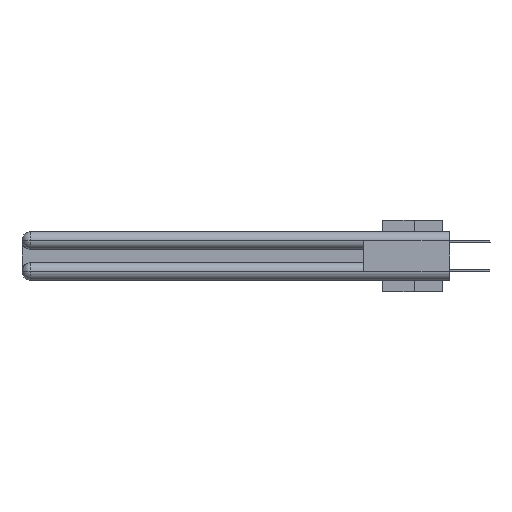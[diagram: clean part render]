
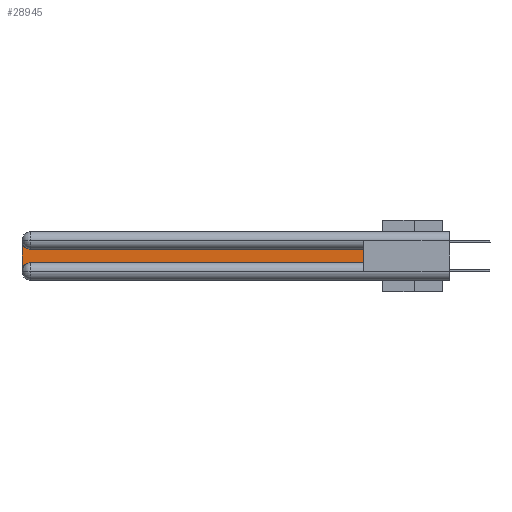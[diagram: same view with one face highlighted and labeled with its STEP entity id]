
A CAD part, left-side view. The second image highlights one B-rep face of the part: STEP entity #28945.
In plain terms, the highlighted planar face has unit normal (-1, 0, 0).
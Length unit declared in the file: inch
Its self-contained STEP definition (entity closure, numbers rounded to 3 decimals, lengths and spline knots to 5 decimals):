
#2207 = CARTESIAN_POINT ( 'NONE',  ( 0.075, 0.6, -0.2175 ) ) ;
#2343 = LINE ( 'NONE', #18107, #22983 ) ;
#2412 = CARTESIAN_POINT ( 'NONE',  ( 0.075, 3., -0.2175 ) ) ;
#2614 = LINE ( 'NONE', #2412, #15412 ) ;
#3167 = VERTEX_POINT ( 'NONE', #26577 ) ;
#3244 = ORIENTED_EDGE ( 'NONE', *, *, #26039, .T. ) ;
#3296 = AXIS2_PLACEMENT_3D ( 'NONE', #23964, #34139, #24758 ) ;
#4093 = CARTESIAN_POINT ( 'NONE',  ( 0.075, 2.94, -0.2775 ) ) ;
#6025 = DIRECTION ( 'NONE',  ( 0., 0., -1. ) ) ;
#6674 = DIRECTION ( 'NONE',  ( 0., -1., 0. ) ) ;
#7266 = EDGE_CURVE ( 'NONE', #7863, #25624, #25875, .T. ) ;
#7273 = CARTESIAN_POINT ( 'NONE',  ( 0.075, 0.6, -0.2175 ) ) ;
#7863 = VERTEX_POINT ( 'NONE', #26794 ) ;
#8315 = ORIENTED_EDGE ( 'NONE', *, *, #7266, .T. ) ;
#9007 = PLANE ( 'NONE',  #3296 ) ;
#10725 = VERTEX_POINT ( 'NONE', #28337 ) ;
#12239 = ORIENTED_EDGE ( 'NONE', *, *, #25417, .T. ) ;
#12454 = CARTESIAN_POINT ( 'NONE',  ( 0.075, 0.6, -0.1225 ) ) ;
#12883 = CIRCLE ( 'NONE', #32966, 0.06 ) ;
#15412 = VECTOR ( 'NONE', #6025, 39.37008 ) ;
#15460 = DIRECTION ( 'NONE',  ( 0., 1., 0. ) ) ;
#18107 = CARTESIAN_POINT ( 'NONE',  ( 0.075, 0.6, -0.1225 ) ) ;
#19349 = DIRECTION ( 'NONE',  ( 0., 0., 1. ) ) ;
#19541 = CARTESIAN_POINT ( 'NONE',  ( 0.075, 0.6, -0.2175 ) ) ;
#20164 = VECTOR ( 'NONE', #6674, 39.37008 ) ;
#20597 = VECTOR ( 'NONE', #19349, 39.37008 ) ;
#21730 = CARTESIAN_POINT ( 'NONE',  ( 0.075, 3., -0.0625 ) ) ;
#22905 = EDGE_CURVE ( 'NONE', #39456, #3167, #2343, .T. ) ;
#22983 = VECTOR ( 'NONE', #15460, 39.37008 ) ;
#23942 = EDGE_LOOP ( 'NONE', ( #31187, #12239, #36973, #3244, #8315, #24468 ) ) ;
#23964 = CARTESIAN_POINT ( 'NONE',  ( 0.075, 3., -0.1225 ) ) ;
#24361 = FACE_OUTER_BOUND ( 'NONE', #23942, .T. ) ;
#24468 = ORIENTED_EDGE ( 'NONE', *, *, #27217, .T. ) ;
#24758 = DIRECTION ( 'NONE',  ( 0., 0., -1. ) ) ;
#25417 = EDGE_CURVE ( 'NONE', #3167, #26151, #36777, .T. ) ;
#25538 = EDGE_CURVE ( 'NONE', #26151, #10725, #2614, .T. ) ;
#25624 = VERTEX_POINT ( 'NONE', #2207 ) ;
#25651 = DIRECTION ( 'NONE',  ( 0., 0., -1. ) ) ;
#25875 = LINE ( 'NONE', #7273, #20164 ) ;
#26039 = EDGE_CURVE ( 'NONE', #10725, #7863, #12883, .T. ) ;
#26151 = VERTEX_POINT ( 'NONE', #21730 ) ;
#26577 = CARTESIAN_POINT ( 'NONE',  ( 0.075, 2.94, -0.1225 ) ) ;
#26794 = CARTESIAN_POINT ( 'NONE',  ( 0.075, 2.94, -0.2175 ) ) ;
#27217 = EDGE_CURVE ( 'NONE', #25624, #39456, #31337, .T. ) ;
#28007 = DIRECTION ( 'NONE',  ( 0., 0., -1. ) ) ;
#28337 = CARTESIAN_POINT ( 'NONE',  ( 0.075, 3., -0.2775 ) ) ;
#28945 = ADVANCED_FACE ( 'NONE', ( #24361 ), #9007, .F. ) ;
#31187 = ORIENTED_EDGE ( 'NONE', *, *, #22905, .T. ) ;
#31337 = LINE ( 'NONE', #19541, #20597 ) ;
#32798 = CARTESIAN_POINT ( 'NONE',  ( 0.075, 2.94, -0.0625 ) ) ;
#32913 = AXIS2_PLACEMENT_3D ( 'NONE', #32798, #38649, #25651 ) ;
#32966 = AXIS2_PLACEMENT_3D ( 'NONE', #4093, #33735, #28007 ) ;
#33735 = DIRECTION ( 'NONE',  ( 1., 0., 0. ) ) ;
#34139 = DIRECTION ( 'NONE',  ( 1., 0., 0. ) ) ;
#36777 = CIRCLE ( 'NONE', #32913, 0.06 ) ;
#36973 = ORIENTED_EDGE ( 'NONE', *, *, #25538, .T. ) ;
#38649 = DIRECTION ( 'NONE',  ( 1., 0., 0. ) ) ;
#39456 = VERTEX_POINT ( 'NONE', #12454 ) ;
